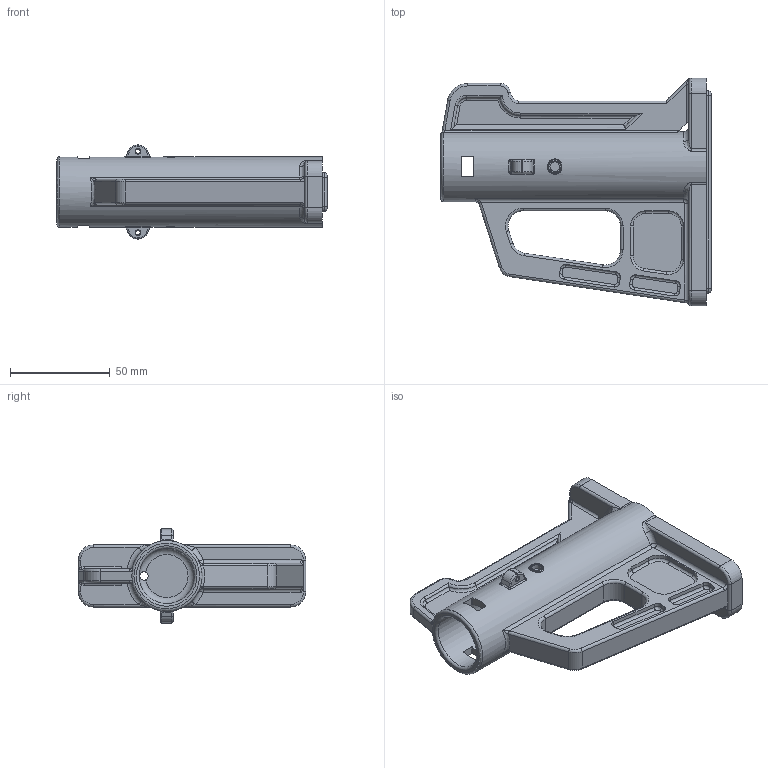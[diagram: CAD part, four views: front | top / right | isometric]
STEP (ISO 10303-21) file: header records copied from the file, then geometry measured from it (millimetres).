
FILE_DESCRIPTION(/* description */ (''),/* implementation_level */ '2;1');
FILE_NAME(/* name */ 'Stock V2.stp',/* time_stamp */ '2021-12-02T15:01:38-06:00',/* author */ ('johne'),/* organization */ (''),/* preprocessor_version */ 'ST-DEVELOPER v18.1',/* originating_system */ 'Autodesk Inventor 2020',/* authorisation */ '');
FILE_SCHEMA (('AUTOMOTIVE_DESIGN { 1 0 10303 214 3 1 1 }'));
Length unit declared in the file: inch
Products named in the file (1): Pho_Spuhr_assembly - Copy
Bounding box: 135.64 x 114.3 x 47.24 mm (x, y, z)
Volume: 126687.2 mm3; surface area: 48689.8 mm2
Topology: 1 solids, 1 shells, 365 faces, 900 edges, 543 vertices
Faces by surface type: cylinder 165, plane 87, bspline 59, torus 54
Full cylindrical faces by diameter (mm): 2.286 x2, 4.2 x2, 4.826 x2, 27.813 x1, 35.433 x1
Entity records: 12459 total; most frequent: CARTESIAN_POINT 3826, DIRECTION 1854, ORIENTED_EDGE 1792, EDGE_CURVE 896, AXIS2_PLACEMENT_3D 746, VERTEX_POINT 543, CIRCLE 390, EDGE_LOOP 389
